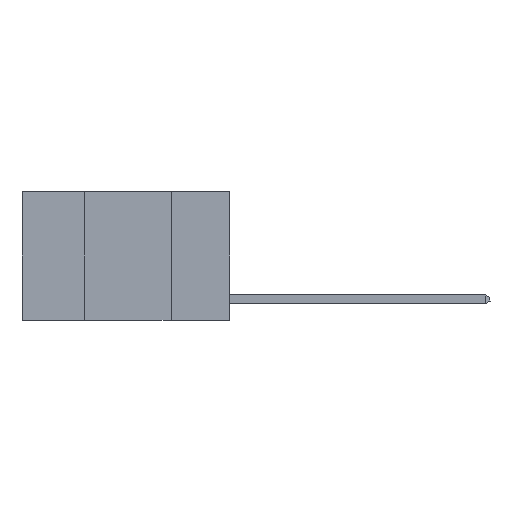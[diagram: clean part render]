
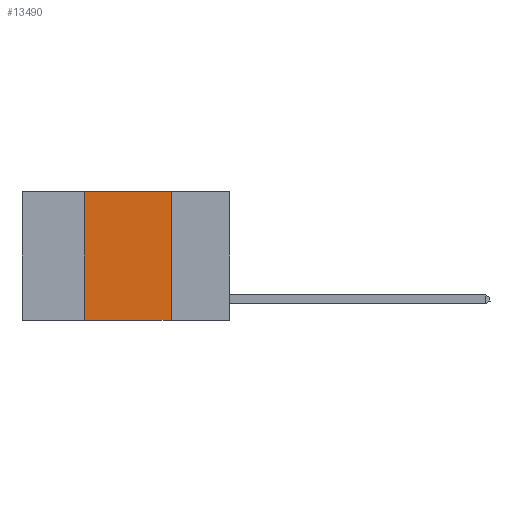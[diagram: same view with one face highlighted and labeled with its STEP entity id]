
A CAD part, left-side view. The second image highlights one B-rep face of the part: STEP entity #13490.
In plain terms, the highlighted planar face has unit normal (-1, 0, 0).
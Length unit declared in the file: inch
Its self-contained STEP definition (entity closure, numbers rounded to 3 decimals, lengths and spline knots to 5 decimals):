
#841 = DIRECTION ( 'NONE',  ( 0., 0., -1. ) ) ;
#2067 = DIRECTION ( 'NONE',  ( 1., 0., 0. ) ) ;
#2244 = VERTEX_POINT ( 'NONE', #18661 ) ;
#2460 = VERTEX_POINT ( 'NONE', #11286 ) ;
#2521 = CARTESIAN_POINT ( 'NONE',  ( 0., 0.17, 0. ) ) ;
#2729 = LINE ( 'NONE', #2521, #20326 ) ;
#3542 = CARTESIAN_POINT ( 'NONE',  ( 0., 0.42, 0. ) ) ;
#4250 = CARTESIAN_POINT ( 'NONE',  ( 0., 0.17, -0.37 ) ) ;
#5246 = VERTEX_POINT ( 'NONE', #4250 ) ;
#5367 = CARTESIAN_POINT ( 'NONE',  ( 0., 0.6, 0. ) ) ;
#5536 = DIRECTION ( 'NONE',  ( 0., 0., 1. ) ) ;
#5626 = DIRECTION ( 'NONE',  ( 0., 0., -1. ) ) ;
#5799 = LINE ( 'NONE', #10637, #16307 ) ;
#9969 = LINE ( 'NONE', #3542, #10535 ) ;
#10535 = VECTOR ( 'NONE', #5536, 39.37008 ) ;
#10550 = CARTESIAN_POINT ( 'NONE',  ( 0., 0.42, -0.37 ) ) ;
#10637 = CARTESIAN_POINT ( 'NONE',  ( 0., 0.6, -0.37 ) ) ;
#11286 = CARTESIAN_POINT ( 'NONE',  ( 0., 0.42, 0. ) ) ;
#13490 = ADVANCED_FACE ( 'NONE', ( #13545 ), #13751, .F. ) ;
#13545 = FACE_OUTER_BOUND ( 'NONE', #14367, .T. ) ;
#13751 = PLANE ( 'NONE',  #13856 ) ;
#13856 = AXIS2_PLACEMENT_3D ( 'NONE', #19969, #2067, #5626 ) ;
#13955 = ORIENTED_EDGE ( 'NONE', *, *, #17707, .F. ) ;
#14253 = EDGE_CURVE ( 'NONE', #2460, #2244, #14873, .T. ) ;
#14367 = EDGE_LOOP ( 'NONE', ( #13955, #15769, #16085, #20750 ) ) ;
#14873 = LINE ( 'NONE', #5367, #19264 ) ;
#14972 = EDGE_CURVE ( 'NONE', #18608, #2460, #9969, .T. ) ;
#15769 = ORIENTED_EDGE ( 'NONE', *, *, #14253, .F. ) ;
#16059 = EDGE_CURVE ( 'NONE', #18608, #5246, #5799, .T. ) ;
#16085 = ORIENTED_EDGE ( 'NONE', *, *, #14972, .F. ) ;
#16307 = VECTOR ( 'NONE', #17173, 39.37008 ) ;
#17173 = DIRECTION ( 'NONE',  ( 0., -1., 0. ) ) ;
#17707 = EDGE_CURVE ( 'NONE', #2244, #5246, #2729, .T. ) ;
#18234 = DIRECTION ( 'NONE',  ( 0., -1., 0. ) ) ;
#18608 = VERTEX_POINT ( 'NONE', #10550 ) ;
#18661 = CARTESIAN_POINT ( 'NONE',  ( 0., 0.17, 0. ) ) ;
#19264 = VECTOR ( 'NONE', #18234, 39.37008 ) ;
#19969 = CARTESIAN_POINT ( 'NONE',  ( 0., 0.6, 0. ) ) ;
#20326 = VECTOR ( 'NONE', #841, 39.37008 ) ;
#20750 = ORIENTED_EDGE ( 'NONE', *, *, #16059, .T. ) ;
